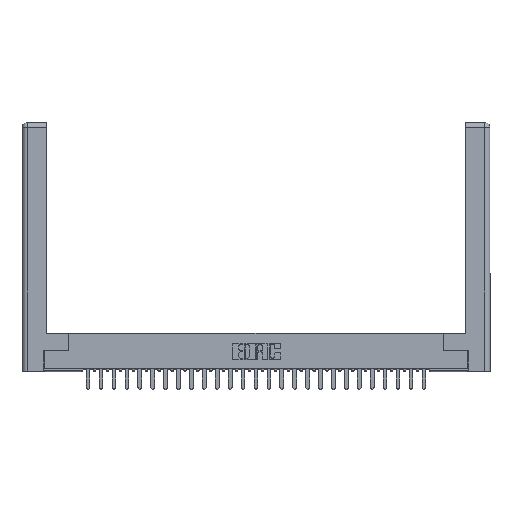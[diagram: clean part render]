
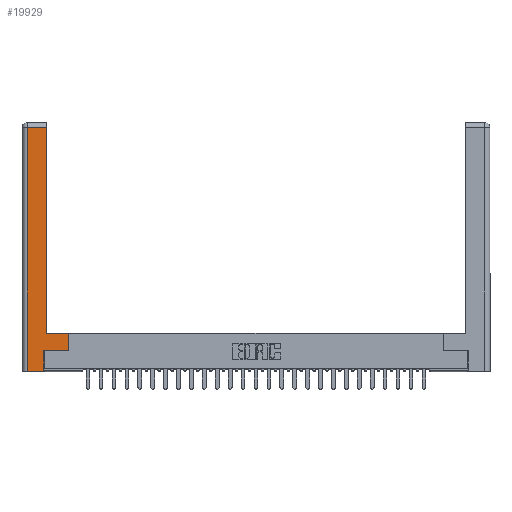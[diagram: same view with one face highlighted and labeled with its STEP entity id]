
A CAD part, top view. The second image highlights one B-rep face of the part: STEP entity #19929.
In plain terms, the highlighted planar face has unit normal (0, 0, 1).
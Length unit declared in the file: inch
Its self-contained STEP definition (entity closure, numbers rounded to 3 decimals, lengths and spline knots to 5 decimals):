
#35 = VECTOR ( 'NONE', #23208, 39.37008 ) ;
#571 = CARTESIAN_POINT ( 'NONE',  ( 0.0615, 2.94, 0. ) ) ;
#753 = VERTEX_POINT ( 'NONE', #15543 ) ;
#997 = CARTESIAN_POINT ( 'NONE',  ( 0.295, 2.94, 0. ) ) ;
#1199 = LINE ( 'NONE', #25912, #4832 ) ;
#1359 = DIRECTION ( 'NONE',  ( 0., 1., 0. ) ) ;
#1443 = LINE ( 'NONE', #6785, #26552 ) ;
#3394 = EDGE_CURVE ( 'NONE', #15039, #12241, #29651, .T. ) ;
#3754 = VECTOR ( 'NONE', #7945, 39.37008 ) ;
#3821 = EDGE_LOOP ( 'NONE', ( #12834, #30035, #32721, #23817, #30089, #29681, #12135, #21576 ) ) ;
#4002 = CARTESIAN_POINT ( 'NONE',  ( 0.295, 0.45, 0. ) ) ;
#4177 = DIRECTION ( 'NONE',  ( -1., 0., 0. ) ) ;
#4816 = VERTEX_POINT ( 'NONE', #18184 ) ;
#4832 = VECTOR ( 'NONE', #26260, 39.37008 ) ;
#5007 = CARTESIAN_POINT ( 'NONE',  ( 0.565, 0.245, 0. ) ) ;
#6297 = CARTESIAN_POINT ( 'NONE',  ( 0.565, 0.245, 0. ) ) ;
#6785 = CARTESIAN_POINT ( 'NONE',  ( 0.565, 0.45, 0. ) ) ;
#7945 = DIRECTION ( 'NONE',  ( 1., 0., 0. ) ) ;
#8701 = CARTESIAN_POINT ( 'NONE',  ( 0.0615, 2.94, 0. ) ) ;
#8922 = CARTESIAN_POINT ( 'NONE',  ( 0.265, 0., 0. ) ) ;
#9017 = CARTESIAN_POINT ( 'NONE',  ( 0., 0., 0. ) ) ;
#9597 = CARTESIAN_POINT ( 'NONE',  ( 0.265, 0.245, 0. ) ) ;
#10190 = FACE_OUTER_BOUND ( 'NONE', #3821, .T. ) ;
#10664 = VECTOR ( 'NONE', #19169, 39.37008 ) ;
#12135 = ORIENTED_EDGE ( 'NONE', *, *, #24072, .T. ) ;
#12215 = CARTESIAN_POINT ( 'NONE',  ( 0.295, 0.45, 0. ) ) ;
#12241 = VERTEX_POINT ( 'NONE', #997 ) ;
#12510 = VERTEX_POINT ( 'NONE', #571 ) ;
#12834 = ORIENTED_EDGE ( 'NONE', *, *, #3394, .T. ) ;
#14555 = DIRECTION ( 'NONE',  ( -1., 0., 0. ) ) ;
#15039 = VERTEX_POINT ( 'NONE', #12215 ) ;
#15543 = CARTESIAN_POINT ( 'NONE',  ( 0.265, 0.245, 0. ) ) ;
#15937 = VERTEX_POINT ( 'NONE', #8922 ) ;
#16954 = DIRECTION ( 'NONE',  ( -1., 0., 0. ) ) ;
#17516 = VERTEX_POINT ( 'NONE', #6297 ) ;
#18184 = CARTESIAN_POINT ( 'NONE',  ( 0.0615, 0., 0. ) ) ;
#18246 = VECTOR ( 'NONE', #14555, 39.37008 ) ;
#19169 = DIRECTION ( 'NONE',  ( 0., -1., 0. ) ) ;
#19929 = ADVANCED_FACE ( 'NONE', ( #10190 ), #22150, .F. ) ;
#20068 = CARTESIAN_POINT ( 'NONE',  ( 0.295, 3., 0. ) ) ;
#20108 = EDGE_CURVE ( 'NONE', #30497, #15039, #23127, .T. ) ;
#21238 = AXIS2_PLACEMENT_3D ( 'NONE', #9017, #29618, #16954 ) ;
#21576 = ORIENTED_EDGE ( 'NONE', *, *, #20108, .T. ) ;
#22150 = PLANE ( 'NONE',  #21238 ) ;
#23124 = VECTOR ( 'NONE', #33005, 39.37008 ) ;
#23127 = LINE ( 'NONE', #4002, #18246 ) ;
#23208 = DIRECTION ( 'NONE',  ( 0., 1., 0. ) ) ;
#23817 = ORIENTED_EDGE ( 'NONE', *, *, #28203, .T. ) ;
#24072 = EDGE_CURVE ( 'NONE', #17516, #30497, #1443, .T. ) ;
#25912 = CARTESIAN_POINT ( 'NONE',  ( 0.265, 0., 0. ) ) ;
#26260 = DIRECTION ( 'NONE',  ( 1., 0., 0. ) ) ;
#26385 = EDGE_CURVE ( 'NONE', #753, #17516, #27273, .T. ) ;
#26552 = VECTOR ( 'NONE', #1359, 39.37008 ) ;
#27209 = VECTOR ( 'NONE', #4177, 39.37008 ) ;
#27273 = LINE ( 'NONE', #5007, #3754 ) ;
#28203 = EDGE_CURVE ( 'NONE', #4816, #15937, #1199, .T. ) ;
#29618 = DIRECTION ( 'NONE',  ( 0., 0., -1. ) ) ;
#29651 = LINE ( 'NONE', #20068, #35 ) ;
#29681 = ORIENTED_EDGE ( 'NONE', *, *, #26385, .T. ) ;
#29735 = EDGE_CURVE ( 'NONE', #12510, #4816, #32528, .T. ) ;
#30035 = ORIENTED_EDGE ( 'NONE', *, *, #31322, .T. ) ;
#30089 = ORIENTED_EDGE ( 'NONE', *, *, #30612, .T. ) ;
#30465 = LINE ( 'NONE', #8701, #27209 ) ;
#30497 = VERTEX_POINT ( 'NONE', #31648 ) ;
#30612 = EDGE_CURVE ( 'NONE', #15937, #753, #31629, .T. ) ;
#31322 = EDGE_CURVE ( 'NONE', #12241, #12510, #30465, .T. ) ;
#31629 = LINE ( 'NONE', #9597, #23124 ) ;
#31648 = CARTESIAN_POINT ( 'NONE',  ( 0.565, 0.45, 0. ) ) ;
#31940 = CARTESIAN_POINT ( 'NONE',  ( 0.0615, 0., 0. ) ) ;
#32528 = LINE ( 'NONE', #31940, #10664 ) ;
#32721 = ORIENTED_EDGE ( 'NONE', *, *, #29735, .T. ) ;
#33005 = DIRECTION ( 'NONE',  ( 0., 1., 0. ) ) ;
